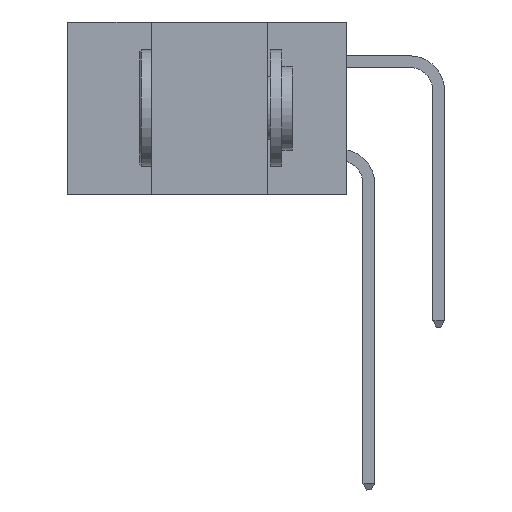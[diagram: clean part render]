
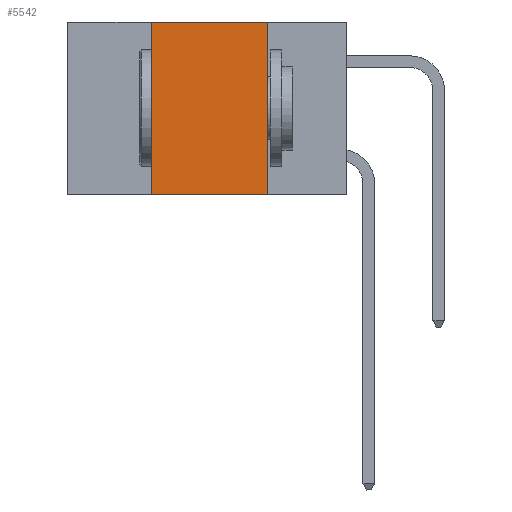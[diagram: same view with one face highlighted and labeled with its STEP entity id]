
A CAD part, left-side view. The second image highlights one B-rep face of the part: STEP entity #5542.
In plain terms, the highlighted planar face has unit normal (-1, 0, 0).
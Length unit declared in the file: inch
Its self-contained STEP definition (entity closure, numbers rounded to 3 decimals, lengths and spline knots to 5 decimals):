
#1151 = DIRECTION ( 'NONE',  ( 0., 0., -1. ) ) ;
#1568 = CARTESIAN_POINT ( 'NONE',  ( 0., 0.17, 0. ) ) ;
#1811 = DIRECTION ( 'NONE',  ( 0., 0., 1. ) ) ;
#2111 = CARTESIAN_POINT ( 'NONE',  ( 0., 0.42, 0. ) ) ;
#2455 = VECTOR ( 'NONE', #19475, 39.37008 ) ;
#2458 = EDGE_CURVE ( 'NONE', #7637, #11085, #16040, .T. ) ;
#4802 = ORIENTED_EDGE ( 'NONE', *, *, #10032, .T. ) ;
#5542 = ADVANCED_FACE ( 'NONE', ( #17464 ), #6226, .F. ) ;
#6226 = PLANE ( 'NONE',  #21565 ) ;
#6621 = ORIENTED_EDGE ( 'NONE', *, *, #20959, .F. ) ;
#7347 = DIRECTION ( 'NONE',  ( 0., -1., 0. ) ) ;
#7395 = VECTOR ( 'NONE', #7347, 39.37008 ) ;
#7574 = CARTESIAN_POINT ( 'NONE',  ( 0., 0.6, 0. ) ) ;
#7637 = VERTEX_POINT ( 'NONE', #1568 ) ;
#8677 = CARTESIAN_POINT ( 'NONE',  ( 0., 0.17, -0.37 ) ) ;
#9637 = DIRECTION ( 'NONE',  ( 0., 0., -1. ) ) ;
#10032 = EDGE_CURVE ( 'NONE', #19082, #11085, #11385, .T. ) ;
#10104 = EDGE_CURVE ( 'NONE', #21065, #7637, #14384, .T. ) ;
#11085 = VERTEX_POINT ( 'NONE', #8677 ) ;
#11385 = LINE ( 'NONE', #19253, #7395 ) ;
#11666 = ORIENTED_EDGE ( 'NONE', *, *, #2458, .F. ) ;
#13614 = CARTESIAN_POINT ( 'NONE',  ( 0., 0.42, 0. ) ) ;
#14384 = LINE ( 'NONE', #7574, #2455 ) ;
#14697 = CARTESIAN_POINT ( 'NONE',  ( 0., 0.17, 0. ) ) ;
#14769 = CARTESIAN_POINT ( 'NONE',  ( 0., 0.6, 0. ) ) ;
#14941 = ORIENTED_EDGE ( 'NONE', *, *, #10104, .F. ) ;
#15412 = CARTESIAN_POINT ( 'NONE',  ( 0., 0.42, -0.37 ) ) ;
#16040 = LINE ( 'NONE', #14697, #19903 ) ;
#17277 = EDGE_LOOP ( 'NONE', ( #11666, #14941, #6621, #4802 ) ) ;
#17464 = FACE_OUTER_BOUND ( 'NONE', #17277, .T. ) ;
#18258 = LINE ( 'NONE', #13614, #18782 ) ;
#18782 = VECTOR ( 'NONE', #1811, 39.37008 ) ;
#19082 = VERTEX_POINT ( 'NONE', #15412 ) ;
#19253 = CARTESIAN_POINT ( 'NONE',  ( 0., 0.6, -0.37 ) ) ;
#19475 = DIRECTION ( 'NONE',  ( 0., -1., 0. ) ) ;
#19790 = DIRECTION ( 'NONE',  ( 1., 0., 0. ) ) ;
#19903 = VECTOR ( 'NONE', #1151, 39.37008 ) ;
#20959 = EDGE_CURVE ( 'NONE', #19082, #21065, #18258, .T. ) ;
#21065 = VERTEX_POINT ( 'NONE', #2111 ) ;
#21565 = AXIS2_PLACEMENT_3D ( 'NONE', #14769, #19790, #9637 ) ;
